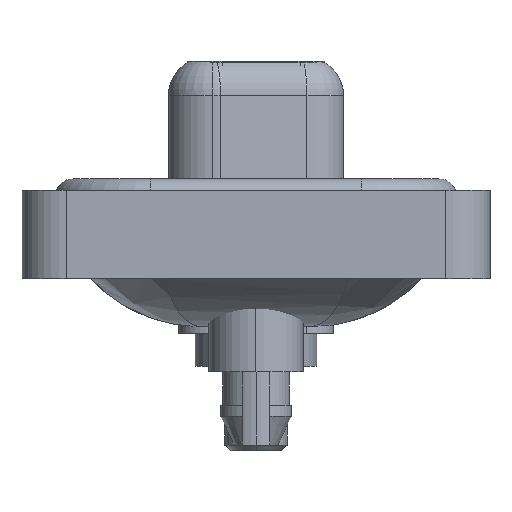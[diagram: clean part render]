
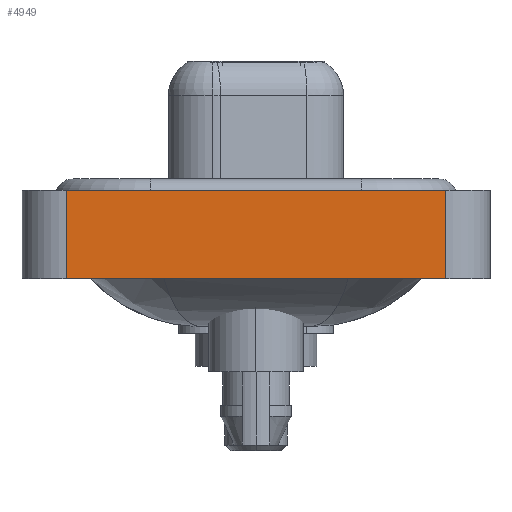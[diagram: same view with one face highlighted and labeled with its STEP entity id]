
A CAD part, left-side view. The second image highlights one B-rep face of the part: STEP entity #4949.
In plain terms, the highlighted planar face has unit normal (-1, 0, 0).
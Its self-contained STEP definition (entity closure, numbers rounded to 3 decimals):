
#89 = VERTEX_POINT ( 'NONE', #16579 ) ;
#255 = VECTOR ( 'NONE', #16398, 1000. ) ;
#481 = DIRECTION ( 'NONE',  ( -1., 0., 0. ) ) ;
#883 = CARTESIAN_POINT ( 'NONE',  ( -7.25, 8.55, 0.4 ) ) ;
#956 = CARTESIAN_POINT ( 'NONE',  ( -7.25, 8.55, -3.6 ) ) ;
#1967 = FACE_OUTER_BOUND ( 'NONE', #2580, .T. ) ;
#2120 = DIRECTION ( 'NONE',  ( 0., -1., 0. ) ) ;
#2580 = EDGE_LOOP ( 'NONE', ( #10465, #12496, #3555, #5836 ) ) ;
#2829 = CARTESIAN_POINT ( 'NONE',  ( -7.25, 8.55, -3.6 ) ) ;
#3555 = ORIENTED_EDGE ( 'NONE', *, *, #9922, .F. ) ;
#4572 = EDGE_CURVE ( 'NONE', #9294, #89, #16505, .T. ) ;
#4949 = ADVANCED_FACE ( 'NONE', ( #1967 ), #11411, .T. ) ;
#5591 = VECTOR ( 'NONE', #2120, 1000. ) ;
#5836 = ORIENTED_EDGE ( 'NONE', *, *, #4572, .T. ) ;
#6767 = LINE ( 'NONE', #2829, #255 ) ;
#6977 = DIRECTION ( 'NONE',  ( 0., 0., 1. ) ) ;
#7874 = CARTESIAN_POINT ( 'NONE',  ( -7.25, -8.55, 0.4 ) ) ;
#8262 = VERTEX_POINT ( 'NONE', #883 ) ;
#8536 = CARTESIAN_POINT ( 'NONE',  ( -7.25, -8.55, -3.6 ) ) ;
#9294 = VERTEX_POINT ( 'NONE', #956 ) ;
#9331 = EDGE_CURVE ( 'NONE', #89, #16114, #13561, .T. ) ;
#9515 = CARTESIAN_POINT ( 'NONE',  ( -7.25, -8.55, -3.6 ) ) ;
#9541 = VECTOR ( 'NONE', #6977, 1000. ) ;
#9823 = CARTESIAN_POINT ( 'NONE',  ( -7.25, -8.55, 0.4 ) ) ;
#9922 = EDGE_CURVE ( 'NONE', #9294, #8262, #6767, .T. ) ;
#10465 = ORIENTED_EDGE ( 'NONE', *, *, #9331, .T. ) ;
#10601 = EDGE_CURVE ( 'NONE', #8262, #16114, #12724, .T. ) ;
#11327 = CARTESIAN_POINT ( 'NONE',  ( -7.25, -8.55, -3.6 ) ) ;
#11411 = PLANE ( 'NONE',  #13099 ) ;
#12496 = ORIENTED_EDGE ( 'NONE', *, *, #10601, .F. ) ;
#12724 = LINE ( 'NONE', #9823, #5591 ) ;
#13099 = AXIS2_PLACEMENT_3D ( 'NONE', #11327, #481, #14136 ) ;
#13561 = LINE ( 'NONE', #9515, #9541 ) ;
#13883 = DIRECTION ( 'NONE',  ( 0., -1., 0. ) ) ;
#14136 = DIRECTION ( 'NONE',  ( 0., 0., 1. ) ) ;
#14476 = VECTOR ( 'NONE', #13883, 1000. ) ;
#16114 = VERTEX_POINT ( 'NONE', #7874 ) ;
#16398 = DIRECTION ( 'NONE',  ( 0., 0., 1. ) ) ;
#16505 = LINE ( 'NONE', #8536, #14476 ) ;
#16579 = CARTESIAN_POINT ( 'NONE',  ( -7.25, -8.55, -3.6 ) ) ;
